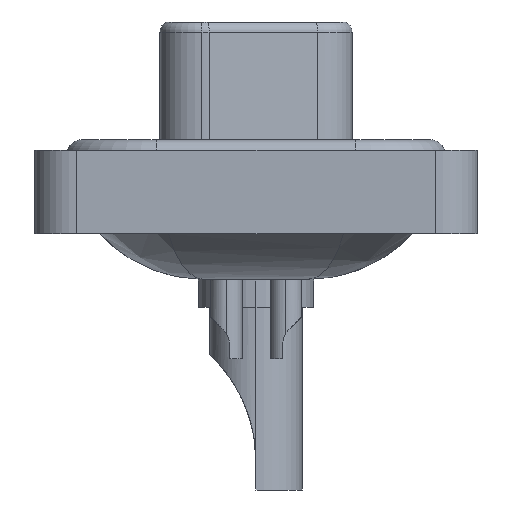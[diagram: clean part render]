
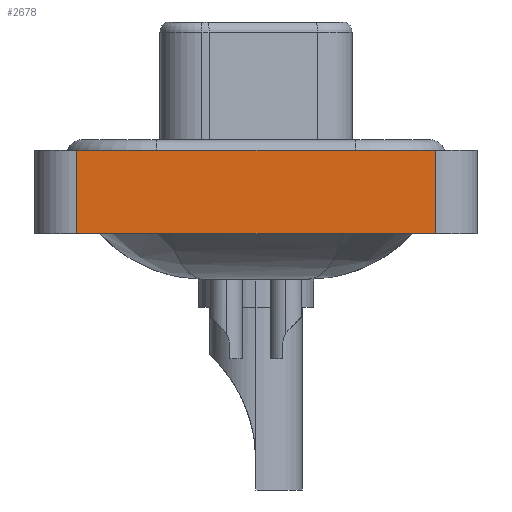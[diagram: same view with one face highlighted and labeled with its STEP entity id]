
A CAD part, left-side view. The second image highlights one B-rep face of the part: STEP entity #2678.
In plain terms, the highlighted planar face has unit normal (-1, 0, 0).
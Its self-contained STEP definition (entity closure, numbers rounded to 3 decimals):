
#85 = EDGE_CURVE ( 'NONE', #5521, #5895, #1119, .T. ) ;
#164 = LINE ( 'NONE', #5708, #11747 ) ;
#390 = LINE ( 'NONE', #3212, #13283 ) ;
#1119 = LINE ( 'NONE', #9378, #9795 ) ;
#1673 = FACE_OUTER_BOUND ( 'NONE', #11451, .T. ) ;
#1807 = DIRECTION ( 'NONE',  ( 0., 0., 1. ) ) ;
#1837 = EDGE_CURVE ( 'NONE', #14432, #5895, #390, .T. ) ;
#2033 = DIRECTION ( 'NONE',  ( 0., -1., 0. ) ) ;
#2678 = ADVANCED_FACE ( 'NONE', ( #1673 ), #11289, .T. ) ;
#3212 = CARTESIAN_POINT ( 'NONE',  ( -7.25, -8.55, 0.4 ) ) ;
#3563 = CARTESIAN_POINT ( 'NONE',  ( -7.25, -8.55, -3.6 ) ) ;
#4226 = VERTEX_POINT ( 'NONE', #5881 ) ;
#5521 = VERTEX_POINT ( 'NONE', #5884 ) ;
#5708 = CARTESIAN_POINT ( 'NONE',  ( -7.25, 8.55, -3.6 ) ) ;
#5858 = DIRECTION ( 'NONE',  ( -1., 0., 0. ) ) ;
#5881 = CARTESIAN_POINT ( 'NONE',  ( -7.25, 8.55, -3.6 ) ) ;
#5884 = CARTESIAN_POINT ( 'NONE',  ( -7.25, -8.55, -3.6 ) ) ;
#5895 = VERTEX_POINT ( 'NONE', #13991 ) ;
#6646 = LINE ( 'NONE', #3563, #13515 ) ;
#7469 = ORIENTED_EDGE ( 'NONE', *, *, #85, .T. ) ;
#7590 = ORIENTED_EDGE ( 'NONE', *, *, #14666, .T. ) ;
#7976 = EDGE_CURVE ( 'NONE', #4226, #14432, #164, .T. ) ;
#8914 = AXIS2_PLACEMENT_3D ( 'NONE', #12462, #5858, #16801 ) ;
#9378 = CARTESIAN_POINT ( 'NONE',  ( -7.25, -8.55, -3.6 ) ) ;
#9607 = ORIENTED_EDGE ( 'NONE', *, *, #7976, .F. ) ;
#9795 = VECTOR ( 'NONE', #12344, 1000. ) ;
#11261 = CARTESIAN_POINT ( 'NONE',  ( -7.25, 8.55, 0.4 ) ) ;
#11289 = PLANE ( 'NONE',  #8914 ) ;
#11451 = EDGE_LOOP ( 'NONE', ( #7469, #11867, #9607, #7590 ) ) ;
#11747 = VECTOR ( 'NONE', #1807, 1000. ) ;
#11867 = ORIENTED_EDGE ( 'NONE', *, *, #1837, .F. ) ;
#12344 = DIRECTION ( 'NONE',  ( 0., 0., 1. ) ) ;
#12462 = CARTESIAN_POINT ( 'NONE',  ( -7.25, -8.55, -3.6 ) ) ;
#13283 = VECTOR ( 'NONE', #2033, 1000. ) ;
#13347 = DIRECTION ( 'NONE',  ( 0., -1., 0. ) ) ;
#13515 = VECTOR ( 'NONE', #13347, 1000. ) ;
#13991 = CARTESIAN_POINT ( 'NONE',  ( -7.25, -8.55, 0.4 ) ) ;
#14432 = VERTEX_POINT ( 'NONE', #11261 ) ;
#14666 = EDGE_CURVE ( 'NONE', #4226, #5521, #6646, .T. ) ;
#16801 = DIRECTION ( 'NONE',  ( 0., 0., 1. ) ) ;
